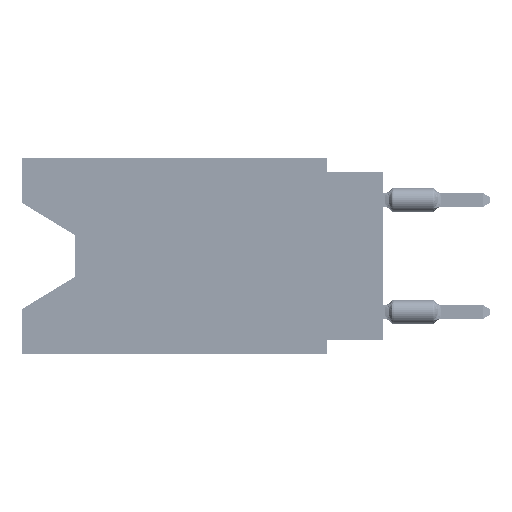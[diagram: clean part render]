
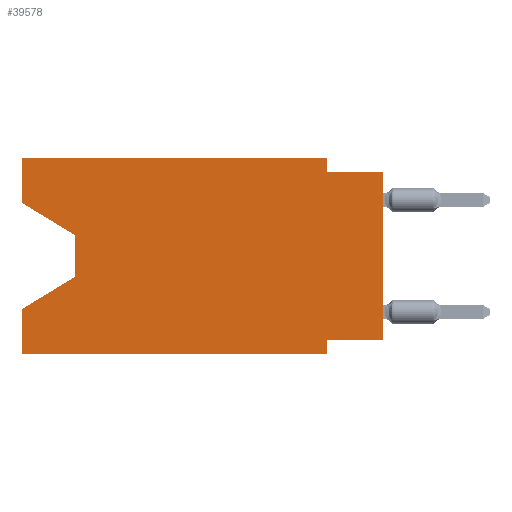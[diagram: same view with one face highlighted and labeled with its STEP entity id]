
A CAD part, left-side view. The second image highlights one B-rep face of the part: STEP entity #39578.
In plain terms, the highlighted planar face has unit normal (-1, 0, 0).
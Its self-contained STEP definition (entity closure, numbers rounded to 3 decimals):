
#3 = ORIENTED_EDGE ( 'NONE', *, *, #37801, .F. ) ;
#1908 = LINE ( 'NONE', #71536, #61894 ) ;
#3747 = EDGE_CURVE ( 'NONE', #6463, #67327, #49806, .T. ) ;
#5677 = ORIENTED_EDGE ( 'NONE', *, *, #110803, .T. ) ;
#6463 = VERTEX_POINT ( 'NONE', #30356 ) ;
#9213 = VERTEX_POINT ( 'NONE', #74753 ) ;
#9811 = LINE ( 'NONE', #105670, #80448 ) ;
#11269 = PLANE ( 'NONE',  #81308 ) ;
#11345 = DIRECTION ( 'NONE',  ( 0., -0.855, -0.519 ) ) ;
#11828 = DIRECTION ( 'NONE',  ( 1., 0., 0. ) ) ;
#12475 = CARTESIAN_POINT ( 'NONE',  ( 0., 16.383, -2.038 ) ) ;
#15691 = DIRECTION ( 'NONE',  ( 0., 0., 1. ) ) ;
#16814 = VERTEX_POINT ( 'NONE', #111780 ) ;
#16923 = ORIENTED_EDGE ( 'NONE', *, *, #68694, .F. ) ;
#17029 = ORIENTED_EDGE ( 'NONE', *, *, #77375, .F. ) ;
#19180 = CARTESIAN_POINT ( 'NONE',  ( 0., 16.383, -8.89 ) ) ;
#19931 = VERTEX_POINT ( 'NONE', #33588 ) ;
#20406 = DIRECTION ( 'NONE',  ( 0., 0., -1. ) ) ;
#21001 = EDGE_CURVE ( 'NONE', #16814, #9213, #85012, .T. ) ;
#21677 = ORIENTED_EDGE ( 'NONE', *, *, #37818, .F. ) ;
#22254 = CARTESIAN_POINT ( 'NONE',  ( 0., 2.54, 0. ) ) ;
#23155 = LINE ( 'NONE', #110440, #105067 ) ;
#23722 = CARTESIAN_POINT ( 'NONE',  ( 0., 16.383, -8.89 ) ) ;
#24049 = ORIENTED_EDGE ( 'NONE', *, *, #40356, .F. ) ;
#25083 = CARTESIAN_POINT ( 'NONE',  ( 0., 0., -0.635 ) ) ;
#26183 = LINE ( 'NONE', #40434, #84186 ) ;
#27052 = CARTESIAN_POINT ( 'NONE',  ( 0., 16.383, -2.038 ) ) ;
#29805 = ORIENTED_EDGE ( 'NONE', *, *, #61821, .F. ) ;
#30356 = CARTESIAN_POINT ( 'NONE',  ( 0., 13.97, -5.385 ) ) ;
#30874 = CARTESIAN_POINT ( 'NONE',  ( 0., 16.383, 0. ) ) ;
#31367 = VERTEX_POINT ( 'NONE', #85508 ) ;
#32584 = EDGE_CURVE ( 'NONE', #75850, #31367, #46706, .T. ) ;
#33588 = CARTESIAN_POINT ( 'NONE',  ( 0., 2.54, -8.89 ) ) ;
#34939 = LINE ( 'NONE', #78905, #75065 ) ;
#37801 = EDGE_CURVE ( 'NONE', #107742, #19931, #110266, .T. ) ;
#37818 = EDGE_CURVE ( 'NONE', #9213, #101854, #103258, .T. ) ;
#38174 = VECTOR ( 'NONE', #39923, 1000. ) ;
#38493 = VECTOR ( 'NONE', #58505, 1000. ) ;
#39380 = ORIENTED_EDGE ( 'NONE', *, *, #3747, .T. ) ;
#39578 = ADVANCED_FACE ( 'NONE', ( #63205 ), #11269, .F. ) ;
#39923 = DIRECTION ( 'NONE',  ( 0., 0., -1. ) ) ;
#40356 = EDGE_CURVE ( 'NONE', #57721, #16814, #83399, .T. ) ;
#40434 = CARTESIAN_POINT ( 'NONE',  ( 0., 16.383, 0. ) ) ;
#45162 = DIRECTION ( 'NONE',  ( 0., 0., 1. ) ) ;
#46706 = LINE ( 'NONE', #12475, #77888 ) ;
#47291 = VERTEX_POINT ( 'NONE', #19180 ) ;
#48983 = ORIENTED_EDGE ( 'NONE', *, *, #50834, .T. ) ;
#49806 = LINE ( 'NONE', #102884, #90392 ) ;
#50834 = EDGE_CURVE ( 'NONE', #47291, #19931, #87056, .T. ) ;
#53166 = DIRECTION ( 'NONE',  ( 0., 0., -1. ) ) ;
#57721 = VERTEX_POINT ( 'NONE', #78398 ) ;
#58505 = DIRECTION ( 'NONE',  ( 0., -1., 0. ) ) ;
#59124 = VECTOR ( 'NONE', #75491, 1000. ) ;
#61821 = EDGE_CURVE ( 'NONE', #103880, #107742, #1908, .T. ) ;
#61894 = VECTOR ( 'NONE', #106334, 1000. ) ;
#63205 = FACE_OUTER_BOUND ( 'NONE', #92256, .T. ) ;
#67327 = VERTEX_POINT ( 'NONE', #98094 ) ;
#68694 = EDGE_CURVE ( 'NONE', #47291, #67327, #26183, .T. ) ;
#71536 = CARTESIAN_POINT ( 'NONE',  ( 0., 0., -8.255 ) ) ;
#72271 = VECTOR ( 'NONE', #72575, 1000. ) ;
#72575 = DIRECTION ( 'NONE',  ( 0., -1., 0. ) ) ;
#73467 = ORIENTED_EDGE ( 'NONE', *, *, #32584, .T. ) ;
#73934 = CARTESIAN_POINT ( 'NONE',  ( 0., 0., -8.255 ) ) ;
#74753 = CARTESIAN_POINT ( 'NONE',  ( 0., 2.54, -0.635 ) ) ;
#74932 = CARTESIAN_POINT ( 'NONE',  ( 0., 2.54, -8.89 ) ) ;
#75065 = VECTOR ( 'NONE', #53166, 1000. ) ;
#75491 = DIRECTION ( 'NONE',  ( 0., 0., -1. ) ) ;
#75850 = VERTEX_POINT ( 'NONE', #27052 ) ;
#77375 = EDGE_CURVE ( 'NONE', #75850, #57721, #23155, .T. ) ;
#77888 = VECTOR ( 'NONE', #11345, 1000. ) ;
#78398 = CARTESIAN_POINT ( 'NONE',  ( 0., 16.383, 0. ) ) ;
#78905 = CARTESIAN_POINT ( 'NONE',  ( 0., 13.97, -3.505 ) ) ;
#80448 = VECTOR ( 'NONE', #45162, 1000. ) ;
#81308 = AXIS2_PLACEMENT_3D ( 'NONE', #98584, #11828, #20406 ) ;
#83399 = LINE ( 'NONE', #30874, #72271 ) ;
#84186 = VECTOR ( 'NONE', #95826, 1000. ) ;
#84337 = EDGE_CURVE ( 'NONE', #103880, #101854, #9811, .T. ) ;
#84501 = CARTESIAN_POINT ( 'NONE',  ( 0., 0., -0.635 ) ) ;
#85012 = LINE ( 'NONE', #22254, #38174 ) ;
#85508 = CARTESIAN_POINT ( 'NONE',  ( 0., 13.97, -3.505 ) ) ;
#87056 = LINE ( 'NONE', #23722, #38493 ) ;
#90392 = VECTOR ( 'NONE', #111448, 1000. ) ;
#92256 = EDGE_LOOP ( 'NONE', ( #73467, #5677, #39380, #16923, #48983, #3, #29805, #101334, #21677, #100248, #24049, #17029 ) ) ;
#95826 = DIRECTION ( 'NONE',  ( 0., 0., 1. ) ) ;
#98094 = CARTESIAN_POINT ( 'NONE',  ( 0., 16.383, -6.852 ) ) ;
#98584 = CARTESIAN_POINT ( 'NONE',  ( 0., 16.383, 0. ) ) ;
#99441 = DIRECTION ( 'NONE',  ( 0., -1., 0. ) ) ;
#100248 = ORIENTED_EDGE ( 'NONE', *, *, #21001, .F. ) ;
#101334 = ORIENTED_EDGE ( 'NONE', *, *, #84337, .T. ) ;
#101854 = VERTEX_POINT ( 'NONE', #84501 ) ;
#102884 = CARTESIAN_POINT ( 'NONE',  ( 0., 13.97, -5.385 ) ) ;
#103258 = LINE ( 'NONE', #25083, #110143 ) ;
#103880 = VERTEX_POINT ( 'NONE', #73934 ) ;
#105067 = VECTOR ( 'NONE', #15691, 1000. ) ;
#105670 = CARTESIAN_POINT ( 'NONE',  ( 0., 0., 0. ) ) ;
#106334 = DIRECTION ( 'NONE',  ( 0., 1., 0. ) ) ;
#107742 = VERTEX_POINT ( 'NONE', #112099 ) ;
#110143 = VECTOR ( 'NONE', #99441, 1000. ) ;
#110266 = LINE ( 'NONE', #74932, #59124 ) ;
#110440 = CARTESIAN_POINT ( 'NONE',  ( 0., 16.383, 0. ) ) ;
#110803 = EDGE_CURVE ( 'NONE', #31367, #6463, #34939, .T. ) ;
#111448 = DIRECTION ( 'NONE',  ( 0., 0.855, -0.519 ) ) ;
#111780 = CARTESIAN_POINT ( 'NONE',  ( 0., 2.54, 0. ) ) ;
#112099 = CARTESIAN_POINT ( 'NONE',  ( 0., 2.54, -8.255 ) ) ;
